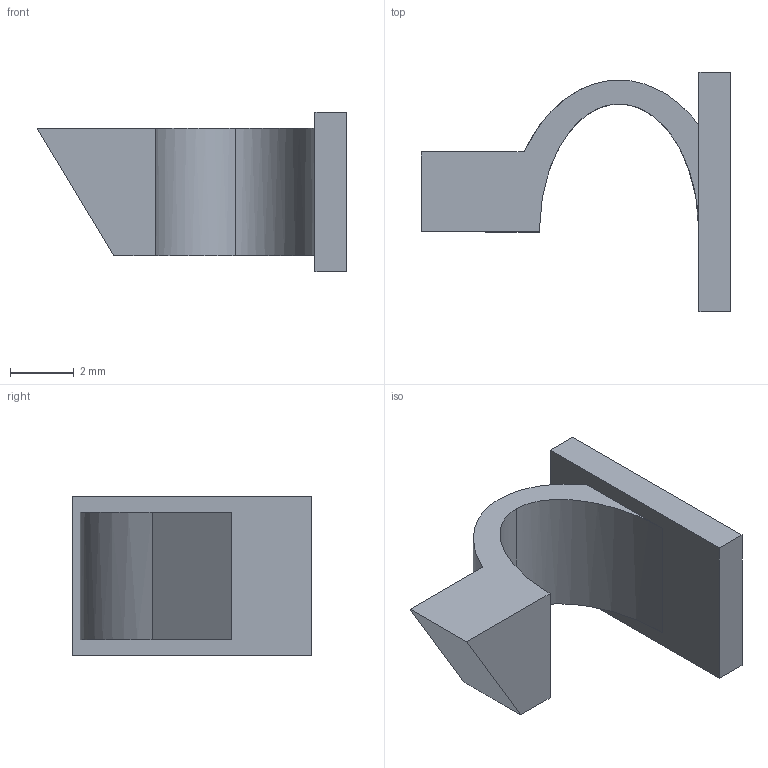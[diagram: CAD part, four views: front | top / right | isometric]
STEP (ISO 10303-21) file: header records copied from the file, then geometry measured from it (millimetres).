
FILE_DESCRIPTION (( 'STEP AP203' ), '1' );
FILE_NAME ('Lock.STEP', '2013-11-14T05:09:33', ( '' ), ( '' ), 'SwSTEP 2.0', 'SolidWorks 2013', '' );
FILE_SCHEMA (( 'CONFIG_CONTROL_DESIGN' ));
Length unit declared in the file: millimetre
Products named in the file (1): Lock
Bounding box: 9.7 x 7.5 x 5 mm (x, y, z)
Volume: 86.7 mm3; surface area: 210.2 mm2
Topology: 1 solids, 1 shells, 15 faces, 36 edges, 24 vertices
Faces by surface type: plane 11, bspline 4
Entity records: 519 total; most frequent: CARTESIAN_POINT 128, ORIENTED_EDGE 72, DIRECTION 52, EDGE_CURVE 36, LINE 28, VECTOR 28, VERTEX_POINT 24, EDGE_LOOP 16
